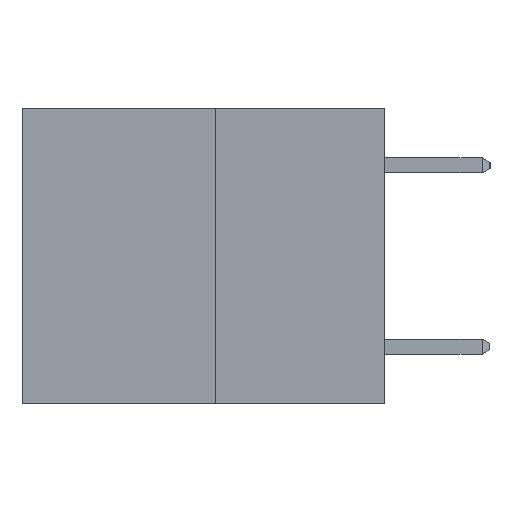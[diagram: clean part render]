
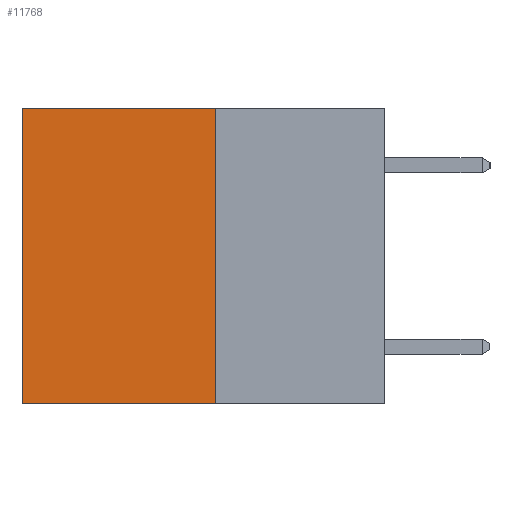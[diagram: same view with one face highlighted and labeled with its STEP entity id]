
A CAD part, left-side view. The second image highlights one B-rep face of the part: STEP entity #11768.
In plain terms, the highlighted planar face has unit normal (-1, 0, 0).
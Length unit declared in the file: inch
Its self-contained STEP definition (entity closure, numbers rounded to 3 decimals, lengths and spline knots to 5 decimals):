
#289 = VECTOR ( 'NONE', #6741, 39.37008 ) ;
#471 = ORIENTED_EDGE ( 'NONE', *, *, #615, .F. ) ;
#615 = EDGE_CURVE ( 'NONE', #1429, #11784, #11607, .T. ) ;
#894 = CARTESIAN_POINT ( 'NONE',  ( 0.3165, 0.28, -0.49 ) ) ;
#1395 = EDGE_CURVE ( 'NONE', #11784, #7934, #8090, .T. ) ;
#1429 = VERTEX_POINT ( 'NONE', #6124 ) ;
#1862 = EDGE_CURVE ( 'NONE', #7436, #7934, #7345, .T. ) ;
#2037 = CARTESIAN_POINT ( 'NONE',  ( 0.3165, 0.6, -0.49 ) ) ;
#2089 = CARTESIAN_POINT ( 'NONE',  ( 0.3165, 0.28, -0.49 ) ) ;
#2099 = EDGE_CURVE ( 'NONE', #1429, #7436, #3495, .T. ) ;
#3495 = LINE ( 'NONE', #9267, #10382 ) ;
#3825 = CARTESIAN_POINT ( 'NONE',  ( 0.3165, 0.28, -0.49 ) ) ;
#6107 = VECTOR ( 'NONE', #7137, 39.37008 ) ;
#6124 = CARTESIAN_POINT ( 'NONE',  ( 0.3165, 0.28, 0. ) ) ;
#6741 = DIRECTION ( 'NONE',  ( 0., 0., -1. ) ) ;
#7016 = DIRECTION ( 'NONE',  ( 0., 1., 0. ) ) ;
#7137 = DIRECTION ( 'NONE',  ( 0., 0., -1. ) ) ;
#7345 = LINE ( 'NONE', #11973, #6107 ) ;
#7365 = AXIS2_PLACEMENT_3D ( 'NONE', #8677, #9705, #10683 ) ;
#7436 = VERTEX_POINT ( 'NONE', #9122 ) ;
#7934 = VERTEX_POINT ( 'NONE', #2037 ) ;
#8090 = LINE ( 'NONE', #2089, #10379 ) ;
#8677 = CARTESIAN_POINT ( 'NONE',  ( 0.3165, 0.28, -0.49 ) ) ;
#8903 = FACE_OUTER_BOUND ( 'NONE', #10501, .T. ) ;
#9105 = ORIENTED_EDGE ( 'NONE', *, *, #2099, .T. ) ;
#9122 = CARTESIAN_POINT ( 'NONE',  ( 0.3165, 0.6, 0. ) ) ;
#9267 = CARTESIAN_POINT ( 'NONE',  ( 0.3165, 0.28, 0. ) ) ;
#9705 = DIRECTION ( 'NONE',  ( 1., 0., 0. ) ) ;
#9987 = ORIENTED_EDGE ( 'NONE', *, *, #1862, .T. ) ;
#10236 = DIRECTION ( 'NONE',  ( 0., 1., 0. ) ) ;
#10379 = VECTOR ( 'NONE', #7016, 39.37008 ) ;
#10382 = VECTOR ( 'NONE', #10236, 39.37008 ) ;
#10501 = EDGE_LOOP ( 'NONE', ( #9987, #11964, #471, #9105 ) ) ;
#10683 = DIRECTION ( 'NONE',  ( 0., 0., -1. ) ) ;
#11607 = LINE ( 'NONE', #894, #289 ) ;
#11638 = PLANE ( 'NONE',  #7365 ) ;
#11768 = ADVANCED_FACE ( 'NONE', ( #8903 ), #11638, .F. ) ;
#11784 = VERTEX_POINT ( 'NONE', #3825 ) ;
#11964 = ORIENTED_EDGE ( 'NONE', *, *, #1395, .F. ) ;
#11973 = CARTESIAN_POINT ( 'NONE',  ( 0.3165, 0.6, -0.49 ) ) ;
